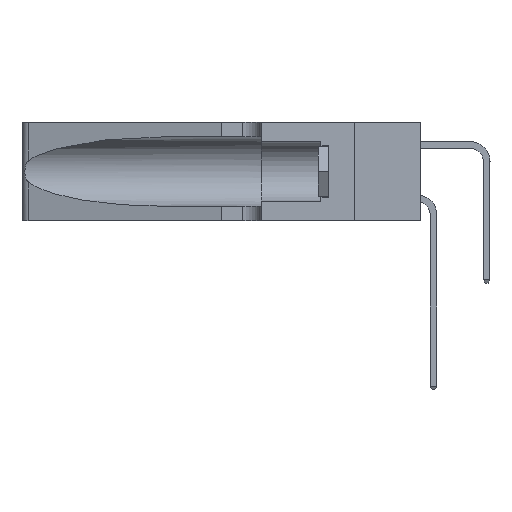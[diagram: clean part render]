
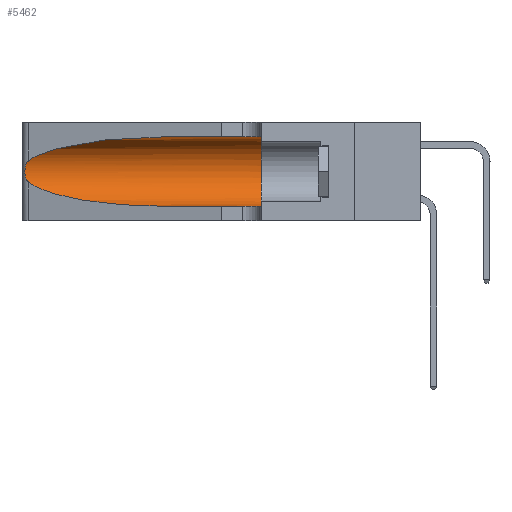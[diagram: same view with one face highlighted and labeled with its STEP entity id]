
A CAD part, left-side view. The second image highlights one B-rep face of the part: STEP entity #5462.
In plain terms, the highlighted cylindrical face has radius 3.308 mm (diameter 6.617 mm), a partial arc.
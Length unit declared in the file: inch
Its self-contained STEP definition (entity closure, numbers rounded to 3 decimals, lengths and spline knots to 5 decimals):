
#415 = DIRECTION ( 'NONE',  ( 0., -1., 0. ) ) ;
#470 = CARTESIAN_POINT ( 'NONE',  ( 0.25487, 1.22718, 0.14631 ) ) ;
#686 = DIRECTION ( 'NONE',  ( 0., 0., 1. ) ) ;
#920 = EDGE_LOOP ( 'NONE', ( #23673, #15252, #4612, #7836, #19314, #21405 ) ) ;
#1170 = CARTESIAN_POINT ( 'NONE',  ( 0.25787, 1.23484, 0.2124 ) ) ;
#3000 = CARTESIAN_POINT ( 'NONE',  ( 0.1305, 1.61858, 0.185 ) ) ;
#3429 = EDGE_CURVE ( 'NONE', #14358, #30708, #21263, .T. ) ;
#3743 = CARTESIAN_POINT ( 'NONE',  ( 0.25555, 1.22993, 0.14849 ) ) ;
#3762 = CARTESIAN_POINT ( 'NONE',  ( 0.25487, 1.22718, 0.14631 ) ) ;
#4612 = ORIENTED_EDGE ( 'NONE', *, *, #3429, .T. ) ;
#5118 = LINE ( 'NONE', #15721, #20948 ) ;
#5462 = ADVANCED_FACE ( 'NONE', ( #21686 ), #28424, .F. ) ;
#5474 = DIRECTION ( 'NONE',  ( 0., -1., 0. ) ) ;
#5762 = DIRECTION ( 'NONE',  ( 0., 1., 0. ) ) ;
#6068 =( BOUNDED_CURVE ( )  B_SPLINE_CURVE ( 3, ( #13728, #13958, #26306, #21198 ),
 .UNSPECIFIED., .F., .T. ) 
 B_SPLINE_CURVE_WITH_KNOTS ( ( 4, 4 ),
 ( 1.5708, 2.84003 ),
 .UNSPECIFIED. ) 
 CURVE ( )  GEOMETRIC_REPRESENTATION_ITEM ( )  RATIONAL_B_SPLINE_CURVE ( ( 1., 0.87, 0.87, 1. ) ) 
 REPRESENTATION_ITEM ( '' )  );
#6639 = VERTEX_POINT ( 'NONE', #25219 ) ;
#6943 = CIRCLE ( 'NONE', #23441, 0.13025 ) ;
#7836 = ORIENTED_EDGE ( 'NONE', *, *, #14877, .T. ) ;
#8564 = CARTESIAN_POINT ( 'NONE',  ( 0.25854, 1.2359, 0.20912 ) ) ;
#8677 = CARTESIAN_POINT ( 'NONE',  ( 0.25639, 1.23184, 0.21858 ) ) ;
#9027 = CARTESIAN_POINT ( 'NONE',  ( 0.25856, 1.23593, 0.16098 ) ) ;
#10144 = LINE ( 'NONE', #15209, #22779 ) ;
#11461 = CARTESIAN_POINT ( 'NONE',  ( 0.25487, 1.22718, 0.22369 ) ) ;
#13620 = AXIS2_PLACEMENT_3D ( 'NONE', #3000, #14743, #14851 ) ;
#13728 = CARTESIAN_POINT ( 'NONE',  ( 0.1305, 0.72297, 0.31525 ) ) ;
#13958 = CARTESIAN_POINT ( 'NONE',  ( 0.18966, 0.96281, 0.31525 ) ) ;
#14358 = VERTEX_POINT ( 'NONE', #470 ) ;
#14456 = EDGE_CURVE ( 'NONE', #6639, #23885, #6068, .T. ) ;
#14743 = DIRECTION ( 'NONE',  ( 0., -1., 0. ) ) ;
#14851 = DIRECTION ( 'NONE',  ( 0., 0., -1. ) ) ;
#14877 = EDGE_CURVE ( 'NONE', #30708, #26028, #10144, .T. ) ;
#15209 = CARTESIAN_POINT ( 'NONE',  ( 0.1305, 1.61858, 0.05475 ) ) ;
#15252 = ORIENTED_EDGE ( 'NONE', *, *, #23088, .T. ) ;
#15350 = VERTEX_POINT ( 'NONE', #24388 ) ;
#15448 = B_SPLINE_CURVE_WITH_KNOTS ( 'NONE', 3,
 ( #11461, #31581, #8677, #1170, #8564, #18965, #21262, #31353, #24172, #9027, #16548, #18179, #3743, #16337 ),
 .UNSPECIFIED., .F., .F.,
 ( 4, 2, 2, 2, 2, 2, 4 ),
 ( 0., 0.00027, 0.00053, 0.00107, 0.0016, 0.00187, 0.00214 ),
 .UNSPECIFIED. ) ;
#15721 = CARTESIAN_POINT ( 'NONE',  ( 0.1305, 1.61858, 0.31525 ) ) ;
#16292 = CARTESIAN_POINT ( 'NONE',  ( 0.25487, 1.22718, 0.22369 ) ) ;
#16337 = CARTESIAN_POINT ( 'NONE',  ( 0.25487, 1.22718, 0.14631 ) ) ;
#16548 = CARTESIAN_POINT ( 'NONE',  ( 0.25789, 1.23486, 0.15765 ) ) ;
#18179 = CARTESIAN_POINT ( 'NONE',  ( 0.25639, 1.23186, 0.15144 ) ) ;
#18307 = EDGE_CURVE ( 'NONE', #6639, #15350, #5118, .T. ) ;
#18965 = CARTESIAN_POINT ( 'NONE',  ( 0.26018, 1.23835, 0.19895 ) ) ;
#19208 = CARTESIAN_POINT ( 'NONE',  ( 0.18966, 0.96281, 0.05475 ) ) ;
#19314 = ORIENTED_EDGE ( 'NONE', *, *, #29772, .F. ) ;
#20246 = CARTESIAN_POINT ( 'NONE',  ( 0.1305, 0.35, 0.05475 ) ) ;
#20948 = VECTOR ( 'NONE', #415, 39.37008 ) ;
#21198 = CARTESIAN_POINT ( 'NONE',  ( 0.25487, 1.22718, 0.22369 ) ) ;
#21262 = CARTESIAN_POINT ( 'NONE',  ( 0.26075, 1.23896, 0.19203 ) ) ;
#21263 =( BOUNDED_CURVE ( )  B_SPLINE_CURVE ( 3, ( #3762, #29277, #19208, #26865 ),
 .UNSPECIFIED., .F., .F. ) 
 B_SPLINE_CURVE_WITH_KNOTS ( ( 4, 4 ),
 ( 3.44316, 4.71239 ),
 .UNSPECIFIED. ) 
 CURVE ( )  GEOMETRIC_REPRESENTATION_ITEM ( )  RATIONAL_B_SPLINE_CURVE ( ( 1., 0.87, 0.87, 1. ) ) 
 REPRESENTATION_ITEM ( '' )  );
#21405 = ORIENTED_EDGE ( 'NONE', *, *, #18307, .F. ) ;
#21686 = FACE_OUTER_BOUND ( 'NONE', #920, .T. ) ;
#22259 = CARTESIAN_POINT ( 'NONE',  ( 0.1305, 0.72297, 0.05475 ) ) ;
#22779 = VECTOR ( 'NONE', #5474, 39.37008 ) ;
#23088 = EDGE_CURVE ( 'NONE', #23885, #14358, #15448, .T. ) ;
#23441 = AXIS2_PLACEMENT_3D ( 'NONE', #23579, #5762, #686 ) ;
#23579 = CARTESIAN_POINT ( 'NONE',  ( 0.1305, 0.35, 0.185 ) ) ;
#23673 = ORIENTED_EDGE ( 'NONE', *, *, #14456, .T. ) ;
#23885 = VERTEX_POINT ( 'NONE', #16292 ) ;
#24172 = CARTESIAN_POINT ( 'NONE',  ( 0.26017, 1.23833, 0.17102 ) ) ;
#24388 = CARTESIAN_POINT ( 'NONE',  ( 0.1305, 0.35, 0.31525 ) ) ;
#25219 = CARTESIAN_POINT ( 'NONE',  ( 0.1305, 0.72297, 0.31525 ) ) ;
#26028 = VERTEX_POINT ( 'NONE', #20246 ) ;
#26306 = CARTESIAN_POINT ( 'NONE',  ( 0.2373, 1.15595, 0.28018 ) ) ;
#26865 = CARTESIAN_POINT ( 'NONE',  ( 0.1305, 0.72297, 0.05475 ) ) ;
#28424 = CYLINDRICAL_SURFACE ( 'NONE', #13620, 0.13025 ) ;
#29277 = CARTESIAN_POINT ( 'NONE',  ( 0.2373, 1.15595, 0.08982 ) ) ;
#29772 = EDGE_CURVE ( 'NONE', #15350, #26028, #6943, .T. ) ;
#30708 = VERTEX_POINT ( 'NONE', #22259 ) ;
#31353 = CARTESIAN_POINT ( 'NONE',  ( 0.26075, 1.23896, 0.178 ) ) ;
#31581 = CARTESIAN_POINT ( 'NONE',  ( 0.25555, 1.22994, 0.2215 ) ) ;
